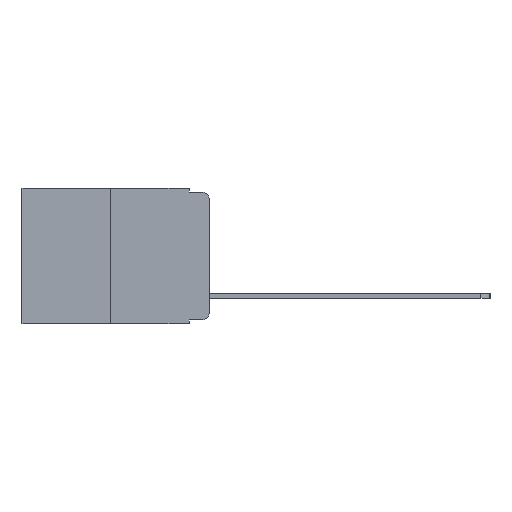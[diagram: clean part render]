
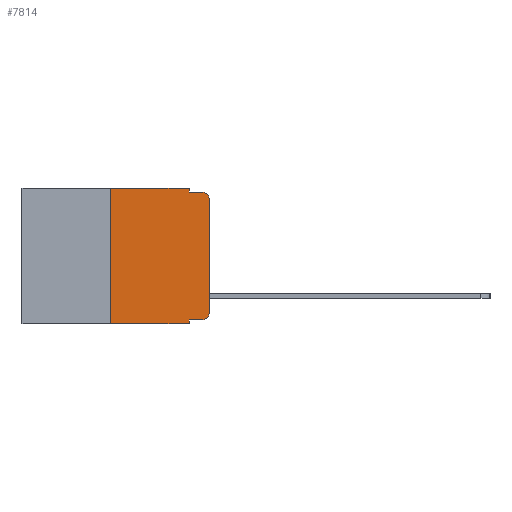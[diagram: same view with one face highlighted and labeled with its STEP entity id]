
A CAD part, left-side view. The second image highlights one B-rep face of the part: STEP entity #7814.
In plain terms, the highlighted planar face has unit normal (-1, 0, 0).
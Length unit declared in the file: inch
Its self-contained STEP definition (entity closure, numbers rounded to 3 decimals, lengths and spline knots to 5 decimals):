
#125 = EDGE_CURVE ( 'NONE', #520, #7527, #9252, .T. ) ;
#270 = DIRECTION ( 'NONE',  ( -1., 0., 0. ) ) ;
#405 = CARTESIAN_POINT ( 'NONE',  ( 0., 0., 0. ) ) ;
#476 = VERTEX_POINT ( 'NONE', #6739 ) ;
#520 = VERTEX_POINT ( 'NONE', #3190 ) ;
#768 = LINE ( 'NONE', #405, #7889 ) ;
#1179 = CARTESIAN_POINT ( 'NONE',  ( 0., 0.473, -0.343 ) ) ;
#1229 = CARTESIAN_POINT ( 'NONE',  ( 0., 0.051, -0.01 ) ) ;
#1279 = CARTESIAN_POINT ( 'NONE',  ( 0., 0.25, -0.343 ) ) ;
#1400 = DIRECTION ( 'NONE',  ( 0., 0., -1. ) ) ;
#1507 = EDGE_CURVE ( 'NONE', #476, #2106, #9359, .T. ) ;
#1768 = ORIENTED_EDGE ( 'NONE', *, *, #11267, .T. ) ;
#1796 = FACE_OUTER_BOUND ( 'NONE', #9291, .T. ) ;
#1829 = DIRECTION ( 'NONE',  ( 0., 0., -1. ) ) ;
#1900 = VERTEX_POINT ( 'NONE', #4286 ) ;
#2071 = VECTOR ( 'NONE', #1829, 39.37008 ) ;
#2078 = EDGE_CURVE ( 'NONE', #1900, #3930, #2949, .T. ) ;
#2088 = VERTEX_POINT ( 'NONE', #10930 ) ;
#2106 = VERTEX_POINT ( 'NONE', #6305 ) ;
#2377 = LINE ( 'NONE', #1179, #4591 ) ;
#2626 = CARTESIAN_POINT ( 'NONE',  ( 0., 0.25, 0. ) ) ;
#2792 = CARTESIAN_POINT ( 'NONE',  ( 0., 0., -0.03 ) ) ;
#2949 = LINE ( 'NONE', #2979, #5699 ) ;
#2979 = CARTESIAN_POINT ( 'NONE',  ( 0., 0.473, 0. ) ) ;
#3064 = EDGE_CURVE ( 'NONE', #2106, #4655, #768, .T. ) ;
#3190 = CARTESIAN_POINT ( 'NONE',  ( 0., 0.051, -0.333 ) ) ;
#3330 = CARTESIAN_POINT ( 'NONE',  ( 0., 0.473, 0. ) ) ;
#3552 = LINE ( 'NONE', #1229, #5994 ) ;
#3714 = AXIS2_PLACEMENT_3D ( 'NONE', #6012, #270, #6901 ) ;
#3875 = CARTESIAN_POINT ( 'NONE',  ( 0., 0.051, -0.343 ) ) ;
#3930 = VERTEX_POINT ( 'NONE', #10259 ) ;
#4286 = CARTESIAN_POINT ( 'NONE',  ( 0., 0.25, 0. ) ) ;
#4312 = DIRECTION ( 'NONE',  ( 0., 0., -1. ) ) ;
#4322 = EDGE_CURVE ( 'NONE', #4655, #2088, #6911, .T. ) ;
#4591 = VECTOR ( 'NONE', #8528, 39.37008 ) ;
#4655 = VERTEX_POINT ( 'NONE', #2792 ) ;
#4939 = EDGE_CURVE ( 'NONE', #5956, #2088, #3552, .T. ) ;
#5032 = ORIENTED_EDGE ( 'NONE', *, *, #1507, .T. ) ;
#5276 = AXIS2_PLACEMENT_3D ( 'NONE', #3330, #6995, #1400 ) ;
#5298 = LINE ( 'NONE', #10403, #9639 ) ;
#5614 = ORIENTED_EDGE ( 'NONE', *, *, #9460, .T. ) ;
#5699 = VECTOR ( 'NONE', #9074, 39.37008 ) ;
#5956 = VERTEX_POINT ( 'NONE', #9037 ) ;
#5994 = VECTOR ( 'NONE', #6857, 39.37008 ) ;
#6012 = CARTESIAN_POINT ( 'NONE',  ( 0., 0.02, -0.03 ) ) ;
#6103 = PLANE ( 'NONE',  #5276 ) ;
#6305 = CARTESIAN_POINT ( 'NONE',  ( 0., 0., -0.313 ) ) ;
#6739 = CARTESIAN_POINT ( 'NONE',  ( 0., 0.02, -0.333 ) ) ;
#6824 = VERTEX_POINT ( 'NONE', #1279 ) ;
#6857 = DIRECTION ( 'NONE',  ( 0., -1., 0. ) ) ;
#6901 = DIRECTION ( 'NONE',  ( 0., 0., -1. ) ) ;
#6911 = CIRCLE ( 'NONE', #3714, 0.02 ) ;
#6995 = DIRECTION ( 'NONE',  ( 1., 0., 0. ) ) ;
#7174 = DIRECTION ( 'NONE',  ( 0., 0., 1. ) ) ;
#7420 = ORIENTED_EDGE ( 'NONE', *, *, #3064, .T. ) ;
#7527 = VERTEX_POINT ( 'NONE', #3875 ) ;
#7706 = CARTESIAN_POINT ( 'NONE',  ( 0., 0.051, -0.333 ) ) ;
#7796 = ORIENTED_EDGE ( 'NONE', *, *, #125, .F. ) ;
#7814 = ADVANCED_FACE ( 'NONE', ( #1796 ), #6103, .F. ) ;
#7889 = VECTOR ( 'NONE', #11118, 39.37008 ) ;
#8109 = ORIENTED_EDGE ( 'NONE', *, *, #4322, .T. ) ;
#8133 = AXIS2_PLACEMENT_3D ( 'NONE', #8248, #8253, #9036 ) ;
#8248 = CARTESIAN_POINT ( 'NONE',  ( 0., 0.02, -0.313 ) ) ;
#8253 = DIRECTION ( 'NONE',  ( -1., 0., 0. ) ) ;
#8472 = EDGE_CURVE ( 'NONE', #6824, #1900, #8883, .T. ) ;
#8489 = LINE ( 'NONE', #7706, #10464 ) ;
#8528 = DIRECTION ( 'NONE',  ( 0., -1., 0. ) ) ;
#8883 = LINE ( 'NONE', #2626, #10833 ) ;
#8991 = ORIENTED_EDGE ( 'NONE', *, *, #8472, .F. ) ;
#9036 = DIRECTION ( 'NONE',  ( 0., 0., -1. ) ) ;
#9037 = CARTESIAN_POINT ( 'NONE',  ( 0., 0.051, -0.01 ) ) ;
#9074 = DIRECTION ( 'NONE',  ( 0., -1., 0. ) ) ;
#9252 = LINE ( 'NONE', #11019, #2071 ) ;
#9291 = EDGE_LOOP ( 'NONE', ( #7420, #8109, #10710, #10189, #9952, #8991, #5614, #7796, #1768, #5032 ) ) ;
#9359 = CIRCLE ( 'NONE', #8133, 0.02 ) ;
#9374 = DIRECTION ( 'NONE',  ( 0., -1., 0. ) ) ;
#9460 = EDGE_CURVE ( 'NONE', #6824, #7527, #2377, .T. ) ;
#9598 = EDGE_CURVE ( 'NONE', #3930, #5956, #5298, .T. ) ;
#9639 = VECTOR ( 'NONE', #4312, 39.37008 ) ;
#9952 = ORIENTED_EDGE ( 'NONE', *, *, #2078, .F. ) ;
#10189 = ORIENTED_EDGE ( 'NONE', *, *, #9598, .F. ) ;
#10259 = CARTESIAN_POINT ( 'NONE',  ( 0., 0.051, 0. ) ) ;
#10403 = CARTESIAN_POINT ( 'NONE',  ( 0., 0.051, 0. ) ) ;
#10464 = VECTOR ( 'NONE', #9374, 39.37008 ) ;
#10710 = ORIENTED_EDGE ( 'NONE', *, *, #4939, .F. ) ;
#10833 = VECTOR ( 'NONE', #7174, 39.37008 ) ;
#10930 = CARTESIAN_POINT ( 'NONE',  ( 0., 0.02, -0.01 ) ) ;
#11019 = CARTESIAN_POINT ( 'NONE',  ( 0., 0.051, 0. ) ) ;
#11118 = DIRECTION ( 'NONE',  ( 0., 0., 1. ) ) ;
#11267 = EDGE_CURVE ( 'NONE', #520, #476, #8489, .T. ) ;
